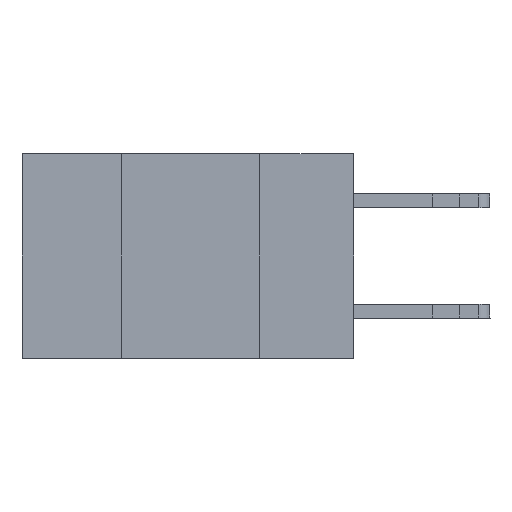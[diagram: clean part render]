
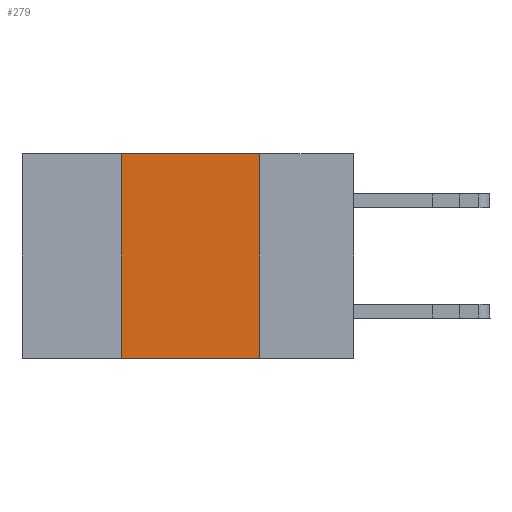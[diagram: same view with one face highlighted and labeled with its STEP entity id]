
A CAD part, left-side view. The second image highlights one B-rep face of the part: STEP entity #279.
In plain terms, the highlighted planar face has unit normal (-1, 0, 0).
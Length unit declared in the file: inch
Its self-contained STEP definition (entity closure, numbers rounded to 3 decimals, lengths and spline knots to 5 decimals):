
#85 = VECTOR ( 'NONE', #30069, 39.37008 ) ;
#96 = VERTEX_POINT ( 'NONE', #6467 ) ;
#241 = EDGE_CURVE ( 'NONE', #12771, #96, #31705, .T. ) ;
#279 = ADVANCED_FACE ( 'NONE', ( #13736 ), #19760, .F. ) ;
#978 = VECTOR ( 'NONE', #22539, 39.37008 ) ;
#2663 = CARTESIAN_POINT ( 'NONE',  ( 0., 0.6, 0. ) ) ;
#3751 = EDGE_CURVE ( 'NONE', #12771, #27808, #18529, .T. ) ;
#6467 = CARTESIAN_POINT ( 'NONE',  ( 0., 0.17, -0.37 ) ) ;
#8843 = LINE ( 'NONE', #15018, #978 ) ;
#9964 = CARTESIAN_POINT ( 'NONE',  ( 0., 0.6, -0.37 ) ) ;
#10352 = CARTESIAN_POINT ( 'NONE',  ( 0., 0.6, 0. ) ) ;
#10392 = EDGE_CURVE ( 'NONE', #13332, #96, #8843, .T. ) ;
#12771 = VERTEX_POINT ( 'NONE', #15129 ) ;
#13134 = ORIENTED_EDGE ( 'NONE', *, *, #241, .T. ) ;
#13332 = VERTEX_POINT ( 'NONE', #16071 ) ;
#13736 = FACE_OUTER_BOUND ( 'NONE', #26691, .T. ) ;
#13875 = ORIENTED_EDGE ( 'NONE', *, *, #10392, .F. ) ;
#15018 = CARTESIAN_POINT ( 'NONE',  ( 0., 0.17, 0. ) ) ;
#15129 = CARTESIAN_POINT ( 'NONE',  ( 0., 0.42, -0.37 ) ) ;
#15290 = DIRECTION ( 'NONE',  ( 1., 0., 0. ) ) ;
#16071 = CARTESIAN_POINT ( 'NONE',  ( 0., 0.17, 0. ) ) ;
#17902 = VECTOR ( 'NONE', #25679, 39.37008 ) ;
#18529 = LINE ( 'NONE', #22905, #85 ) ;
#18978 = DIRECTION ( 'NONE',  ( 0., 0., -1. ) ) ;
#19262 = EDGE_CURVE ( 'NONE', #27808, #13332, #21028, .T. ) ;
#19760 = PLANE ( 'NONE',  #24638 ) ;
#21028 = LINE ( 'NONE', #10352, #17902 ) ;
#22539 = DIRECTION ( 'NONE',  ( 0., 0., -1. ) ) ;
#22905 = CARTESIAN_POINT ( 'NONE',  ( 0., 0.42, 0. ) ) ;
#23137 = CARTESIAN_POINT ( 'NONE',  ( 0., 0.42, 0. ) ) ;
#24638 = AXIS2_PLACEMENT_3D ( 'NONE', #2663, #15290, #18978 ) ;
#25679 = DIRECTION ( 'NONE',  ( 0., -1., 0. ) ) ;
#26265 = VECTOR ( 'NONE', #30140, 39.37008 ) ;
#26691 = EDGE_LOOP ( 'NONE', ( #13875, #26932, #29618, #13134 ) ) ;
#26932 = ORIENTED_EDGE ( 'NONE', *, *, #19262, .F. ) ;
#27808 = VERTEX_POINT ( 'NONE', #23137 ) ;
#29618 = ORIENTED_EDGE ( 'NONE', *, *, #3751, .F. ) ;
#30069 = DIRECTION ( 'NONE',  ( 0., 0., 1. ) ) ;
#30140 = DIRECTION ( 'NONE',  ( 0., -1., 0. ) ) ;
#31705 = LINE ( 'NONE', #9964, #26265 ) ;
